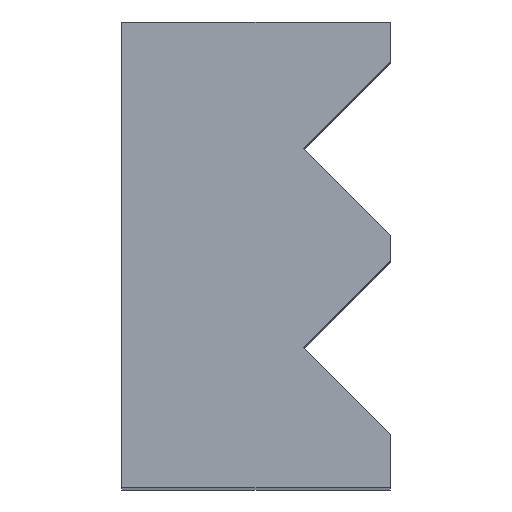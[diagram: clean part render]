
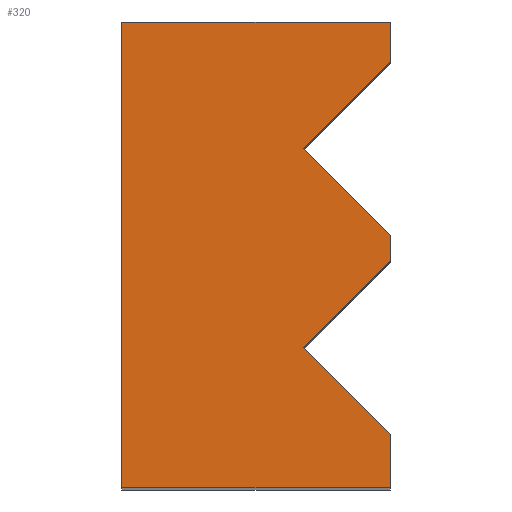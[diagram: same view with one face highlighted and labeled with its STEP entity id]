
A CAD part, top view. The second image highlights one B-rep face of the part: STEP entity #320.
In plain terms, the highlighted planar face has unit normal (0, 0, 1).
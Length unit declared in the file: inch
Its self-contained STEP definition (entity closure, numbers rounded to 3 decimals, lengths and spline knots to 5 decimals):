
#15=LINE('',#487,#49);
#21=LINE('',#498,#55);
#24=LINE('',#504,#58);
#25=LINE('',#508,#59);
#33=LINE('',#521,#67);
#34=LINE('',#525,#68);
#42=LINE('',#538,#76);
#43=LINE('',#540,#77);
#44=LINE('',#541,#78);
#45=LINE('',#542,#79);
#49=VECTOR('',#401,39.37008);
#55=VECTOR('',#409,39.37008);
#58=VECTOR('',#414,39.37008);
#59=VECTOR('',#417,39.37008);
#67=VECTOR('',#427,39.37008);
#68=VECTOR('',#430,39.37008);
#76=VECTOR('',#440,39.37008);
#77=VECTOR('',#443,39.37008);
#78=VECTOR('',#444,39.37008);
#79=VECTOR('',#445,39.37008);
#90=PLANE('',#366);
#110=FACE_OUTER_BOUND('',#130,.T.);
#130=EDGE_LOOP('',(#269,#270,#271,#272,#273,#274,#275,#276,#277,#278));
#157=VERTEX_POINT('',#485);
#158=VERTEX_POINT('',#486);
#162=VERTEX_POINT('',#496);
#164=VERTEX_POINT('',#502);
#165=VERTEX_POINT('',#506);
#166=VERTEX_POINT('',#507);
#170=VERTEX_POINT('',#519);
#171=VERTEX_POINT('',#523);
#172=VERTEX_POINT('',#524);
#176=VERTEX_POINT('',#536);
#187=EDGE_CURVE('',#157,#158,#15,.T.);
#193=EDGE_CURVE('',#158,#162,#21,.T.);
#196=EDGE_CURVE('',#162,#164,#24,.T.);
#197=EDGE_CURVE('',#165,#166,#25,.T.);
#205=EDGE_CURVE('',#166,#170,#33,.T.);
#206=EDGE_CURVE('',#171,#172,#34,.T.);
#214=EDGE_CURVE('',#172,#176,#42,.T.);
#215=EDGE_CURVE('',#165,#164,#43,.T.);
#216=EDGE_CURVE('',#171,#170,#44,.T.);
#217=EDGE_CURVE('',#157,#176,#45,.T.);
#269=ORIENTED_EDGE('',*,*,#196,.T.);
#270=ORIENTED_EDGE('',*,*,#215,.F.);
#271=ORIENTED_EDGE('',*,*,#197,.T.);
#272=ORIENTED_EDGE('',*,*,#205,.T.);
#273=ORIENTED_EDGE('',*,*,#216,.F.);
#274=ORIENTED_EDGE('',*,*,#206,.T.);
#275=ORIENTED_EDGE('',*,*,#214,.T.);
#276=ORIENTED_EDGE('',*,*,#217,.F.);
#277=ORIENTED_EDGE('',*,*,#187,.T.);
#278=ORIENTED_EDGE('',*,*,#193,.T.);
#320=ADVANCED_FACE('',(#110),#90,.F.);
#366=AXIS2_PLACEMENT_3D('',#539,#441,#442);
#401=DIRECTION('',(-1.,0.,0.));
#409=DIRECTION('',(0.,-1.,0.));
#414=DIRECTION('',(1.,0.,0.));
#417=DIRECTION('',(-0.707,0.707,0.));
#427=DIRECTION('',(0.707,0.707,0.));
#430=DIRECTION('',(-0.707,0.707,0.));
#440=DIRECTION('',(0.707,0.707,0.));
#441=DIRECTION('center_axis',(0.,0.,-1.));
#442=DIRECTION('ref_axis',(-1.,0.,0.));
#443=DIRECTION('',(0.,-1.,0.));
#444=DIRECTION('',(0.,-1.,0.));
#445=DIRECTION('',(0.,-1.,0.));
#485=CARTESIAN_POINT('',(-0.3335,0.505,1.25));
#486=CARTESIAN_POINT('',(-0.625,0.505,1.25));
#487=CARTESIAN_POINT('',(-0.3085,0.505,1.25));
#496=CARTESIAN_POINT('',(-0.625,0.,1.25));
#498=CARTESIAN_POINT('',(-0.625,0.,1.25));
#502=CARTESIAN_POINT('',(-0.3335,0.,1.25));
#504=CARTESIAN_POINT('',(-0.32,0.,1.25));
#506=CARTESIAN_POINT('',(-0.3335,0.0575,1.25));
#507=CARTESIAN_POINT('',(-0.428,0.152,1.25));
#508=CARTESIAN_POINT('',(-0.428,0.152,1.25));
#519=CARTESIAN_POINT('',(-0.3335,0.2465,1.25));
#521=CARTESIAN_POINT('',(-0.32,0.26,1.25));
#523=CARTESIAN_POINT('',(-0.3335,0.2735,1.25));
#524=CARTESIAN_POINT('',(-0.428,0.368,1.25));
#525=CARTESIAN_POINT('',(-0.428,0.368,1.25));
#536=CARTESIAN_POINT('',(-0.3335,0.4625,1.25));
#538=CARTESIAN_POINT('',(-0.32,0.476,1.25));
#539=CARTESIAN_POINT('Origin',(-0.625,0.505,1.25));
#540=CARTESIAN_POINT('',(-0.3335,0.505,1.25));
#541=CARTESIAN_POINT('',(-0.3335,0.505,1.25));
#542=CARTESIAN_POINT('',(-0.3335,0.505,1.25));
